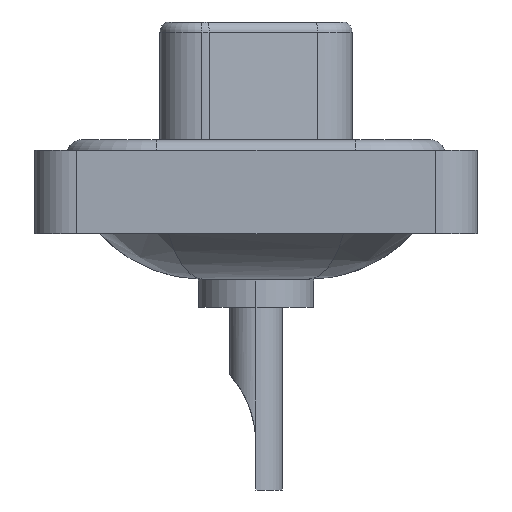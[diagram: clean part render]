
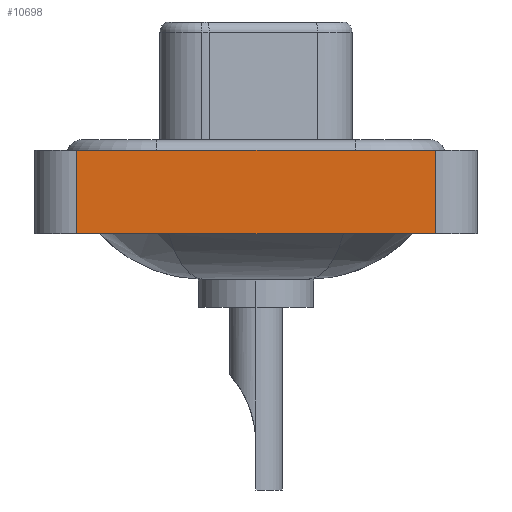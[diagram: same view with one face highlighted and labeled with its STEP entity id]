
A CAD part, left-side view. The second image highlights one B-rep face of the part: STEP entity #10698.
In plain terms, the highlighted planar face has unit normal (-1, 0, 0).
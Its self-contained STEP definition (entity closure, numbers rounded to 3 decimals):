
#525 = DIRECTION ( 'NONE',  ( 0., 0., 1. ) ) ;
#642 = VECTOR ( 'NONE', #14244, 1000. ) ;
#873 = VECTOR ( 'NONE', #2751, 1000. ) ;
#998 = CARTESIAN_POINT ( 'NONE',  ( -7.25, -8.55, -3.6 ) ) ;
#1136 = DIRECTION ( 'NONE',  ( 0., -1., 0. ) ) ;
#1210 = LINE ( 'NONE', #4587, #642 ) ;
#1689 = EDGE_LOOP ( 'NONE', ( #10955, #12723, #10535, #12530 ) ) ;
#2751 = DIRECTION ( 'NONE',  ( 0., -1., 0. ) ) ;
#3457 = EDGE_CURVE ( 'NONE', #6559, #10751, #6216, .T. ) ;
#3692 = EDGE_CURVE ( 'NONE', #5860, #6559, #1210, .T. ) ;
#3966 = CARTESIAN_POINT ( 'NONE',  ( -7.25, -8.55, 0.4 ) ) ;
#4197 = DIRECTION ( 'NONE',  ( -1., 0., 0. ) ) ;
#4559 = EDGE_CURVE ( 'NONE', #5696, #10751, #6913, .T. ) ;
#4587 = CARTESIAN_POINT ( 'NONE',  ( -7.25, 8.55, -3.6 ) ) ;
#4988 = FACE_OUTER_BOUND ( 'NONE', #1689, .T. ) ;
#5432 = PLANE ( 'NONE',  #10770 ) ;
#5484 = CARTESIAN_POINT ( 'NONE',  ( -7.25, 8.55, -3.6 ) ) ;
#5696 = VERTEX_POINT ( 'NONE', #7494 ) ;
#5860 = VERTEX_POINT ( 'NONE', #5484 ) ;
#6216 = LINE ( 'NONE', #14622, #873 ) ;
#6559 = VERTEX_POINT ( 'NONE', #11527 ) ;
#6913 = LINE ( 'NONE', #998, #10477 ) ;
#7494 = CARTESIAN_POINT ( 'NONE',  ( -7.25, -8.55, -3.6 ) ) ;
#7969 = LINE ( 'NONE', #13162, #8320 ) ;
#8320 = VECTOR ( 'NONE', #1136, 1000. ) ;
#8705 = EDGE_CURVE ( 'NONE', #5860, #5696, #7969, .T. ) ;
#10257 = DIRECTION ( 'NONE',  ( 0., 0., 1. ) ) ;
#10477 = VECTOR ( 'NONE', #10257, 1000. ) ;
#10535 = ORIENTED_EDGE ( 'NONE', *, *, #3692, .F. ) ;
#10698 = ADVANCED_FACE ( 'NONE', ( #4988 ), #5432, .T. ) ;
#10751 = VERTEX_POINT ( 'NONE', #3966 ) ;
#10770 = AXIS2_PLACEMENT_3D ( 'NONE', #11237, #4197, #525 ) ;
#10955 = ORIENTED_EDGE ( 'NONE', *, *, #4559, .T. ) ;
#11237 = CARTESIAN_POINT ( 'NONE',  ( -7.25, -8.55, -3.6 ) ) ;
#11527 = CARTESIAN_POINT ( 'NONE',  ( -7.25, 8.55, 0.4 ) ) ;
#12530 = ORIENTED_EDGE ( 'NONE', *, *, #8705, .T. ) ;
#12723 = ORIENTED_EDGE ( 'NONE', *, *, #3457, .F. ) ;
#13162 = CARTESIAN_POINT ( 'NONE',  ( -7.25, -8.55, -3.6 ) ) ;
#14244 = DIRECTION ( 'NONE',  ( 0., 0., 1. ) ) ;
#14622 = CARTESIAN_POINT ( 'NONE',  ( -7.25, -8.55, 0.4 ) ) ;
